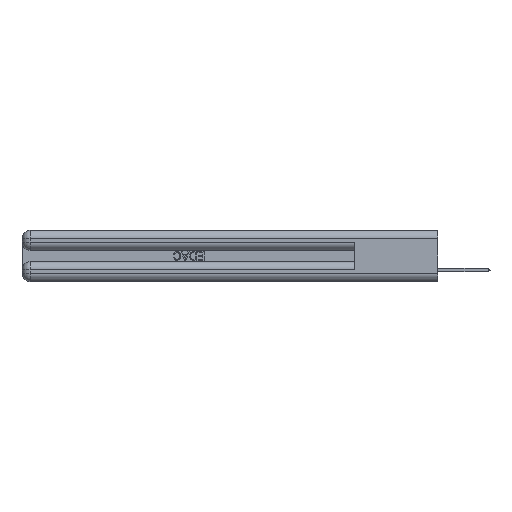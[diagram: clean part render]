
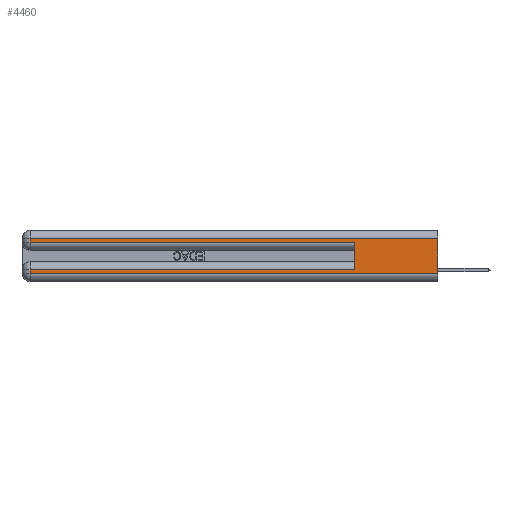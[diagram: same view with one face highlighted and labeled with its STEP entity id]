
A CAD part, left-side view. The second image highlights one B-rep face of the part: STEP entity #4460.
In plain terms, the highlighted planar face has unit normal (-1, 0, 0).
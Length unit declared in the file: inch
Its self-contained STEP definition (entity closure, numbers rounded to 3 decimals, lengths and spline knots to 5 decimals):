
#955 = CARTESIAN_POINT ( 'NONE',  ( 0., 2.94, 0.06 ) ) ;
#1047 = VECTOR ( 'NONE', #7433, 39.37008 ) ;
#1918 = VERTEX_POINT ( 'NONE', #12780 ) ;
#2575 = CARTESIAN_POINT ( 'NONE',  ( 0., 0., 0.085 ) ) ;
#3212 = EDGE_CURVE ( 'NONE', #19215, #30569, #13825, .T. ) ;
#3263 = EDGE_CURVE ( 'NONE', #1918, #7504, #22708, .T. ) ;
#3771 = CARTESIAN_POINT ( 'NONE',  ( 0., 2.94, 0.085 ) ) ;
#4460 = ADVANCED_FACE ( 'NONE', ( #31275 ), #17699, .F. ) ;
#4609 = CARTESIAN_POINT ( 'NONE',  ( 0., 0., 0.37 ) ) ;
#5494 = VECTOR ( 'NONE', #23132, 39.37008 ) ;
#5838 = VECTOR ( 'NONE', #17231, 39.37008 ) ;
#6395 = ORIENTED_EDGE ( 'NONE', *, *, #29933, .T. ) ;
#7119 = VECTOR ( 'NONE', #32649, 39.37008 ) ;
#7433 = DIRECTION ( 'NONE',  ( 0., -1., 0. ) ) ;
#7504 = VERTEX_POINT ( 'NONE', #3771 ) ;
#7667 = CARTESIAN_POINT ( 'NONE',  ( 0., 2.94, 0.37 ) ) ;
#8410 = VERTEX_POINT ( 'NONE', #14242 ) ;
#8619 = EDGE_CURVE ( 'NONE', #17356, #27710, #9027, .T. ) ;
#9027 = LINE ( 'NONE', #19347, #1047 ) ;
#9787 = EDGE_CURVE ( 'NONE', #22203, #27710, #37399, .T. ) ;
#9966 = CARTESIAN_POINT ( 'NONE',  ( 0., 0., 0.31 ) ) ;
#10140 = ORIENTED_EDGE ( 'NONE', *, *, #3212, .T. ) ;
#10824 = EDGE_LOOP ( 'NONE', ( #20897, #33608, #10140, #6395, #31819, #33101, #37631, #12630 ) ) ;
#11378 = CARTESIAN_POINT ( 'NONE',  ( 0., 0., 0.06 ) ) ;
#11544 = EDGE_CURVE ( 'NONE', #1918, #8410, #37450, .T. ) ;
#12114 = EDGE_CURVE ( 'NONE', #22203, #19215, #27170, .T. ) ;
#12409 = CARTESIAN_POINT ( 'NONE',  ( 0., 0., 0.31 ) ) ;
#12630 = ORIENTED_EDGE ( 'NONE', *, *, #8619, .T. ) ;
#12780 = CARTESIAN_POINT ( 'NONE',  ( 0., 0.6, 0.085 ) ) ;
#12832 = DIRECTION ( 'NONE',  ( 1., 0., 0. ) ) ;
#13384 = DIRECTION ( 'NONE',  ( 0., 0., -1. ) ) ;
#13825 = LINE ( 'NONE', #38314, #24988 ) ;
#14132 = VECTOR ( 'NONE', #24063, 39.37008 ) ;
#14134 = CARTESIAN_POINT ( 'NONE',  ( 0., 0., 0.285 ) ) ;
#14242 = CARTESIAN_POINT ( 'NONE',  ( 0., 0.6, 0.285 ) ) ;
#14422 = CARTESIAN_POINT ( 'NONE',  ( 0., 2.94, 0.31 ) ) ;
#17231 = DIRECTION ( 'NONE',  ( 0., 1., 0. ) ) ;
#17356 = VERTEX_POINT ( 'NONE', #955 ) ;
#17699 = PLANE ( 'NONE',  #30834 ) ;
#19215 = VERTEX_POINT ( 'NONE', #14422 ) ;
#19257 = CARTESIAN_POINT ( 'NONE',  ( 0., 0., 0.37 ) ) ;
#19347 = CARTESIAN_POINT ( 'NONE',  ( 0., 0., 0.06 ) ) ;
#20236 = EDGE_CURVE ( 'NONE', #7504, #17356, #35558, .T. ) ;
#20897 = ORIENTED_EDGE ( 'NONE', *, *, #9787, .F. ) ;
#22203 = VERTEX_POINT ( 'NONE', #12409 ) ;
#22708 = LINE ( 'NONE', #2575, #5838 ) ;
#23132 = DIRECTION ( 'NONE',  ( 0., -1., 0. ) ) ;
#24063 = DIRECTION ( 'NONE',  ( 0., 0., -1. ) ) ;
#24988 = VECTOR ( 'NONE', #25976, 39.37008 ) ;
#25589 = LINE ( 'NONE', #14134, #5494 ) ;
#25976 = DIRECTION ( 'NONE',  ( 0., 0., -1. ) ) ;
#26090 = CARTESIAN_POINT ( 'NONE',  ( 0., 2.94, 0.285 ) ) ;
#27170 = LINE ( 'NONE', #9966, #27681 ) ;
#27681 = VECTOR ( 'NONE', #31354, 39.37008 ) ;
#27710 = VERTEX_POINT ( 'NONE', #11378 ) ;
#29933 = EDGE_CURVE ( 'NONE', #30569, #8410, #25589, .T. ) ;
#30569 = VERTEX_POINT ( 'NONE', #26090 ) ;
#30834 = AXIS2_PLACEMENT_3D ( 'NONE', #19257, #12832, #33577 ) ;
#31275 = FACE_OUTER_BOUND ( 'NONE', #10824, .T. ) ;
#31354 = DIRECTION ( 'NONE',  ( 0., 1., 0. ) ) ;
#31812 = VECTOR ( 'NONE', #13384, 39.37008 ) ;
#31819 = ORIENTED_EDGE ( 'NONE', *, *, #11544, .F. ) ;
#32527 = CARTESIAN_POINT ( 'NONE',  ( 0., 0.6, 0.145 ) ) ;
#32649 = DIRECTION ( 'NONE',  ( 0., 0., 1. ) ) ;
#33101 = ORIENTED_EDGE ( 'NONE', *, *, #3263, .T. ) ;
#33577 = DIRECTION ( 'NONE',  ( 0., 0., -1. ) ) ;
#33608 = ORIENTED_EDGE ( 'NONE', *, *, #12114, .T. ) ;
#35558 = LINE ( 'NONE', #7667, #14132 ) ;
#37399 = LINE ( 'NONE', #4609, #31812 ) ;
#37450 = LINE ( 'NONE', #32527, #7119 ) ;
#37631 = ORIENTED_EDGE ( 'NONE', *, *, #20236, .T. ) ;
#38314 = CARTESIAN_POINT ( 'NONE',  ( 0., 2.94, 0.37 ) ) ;
